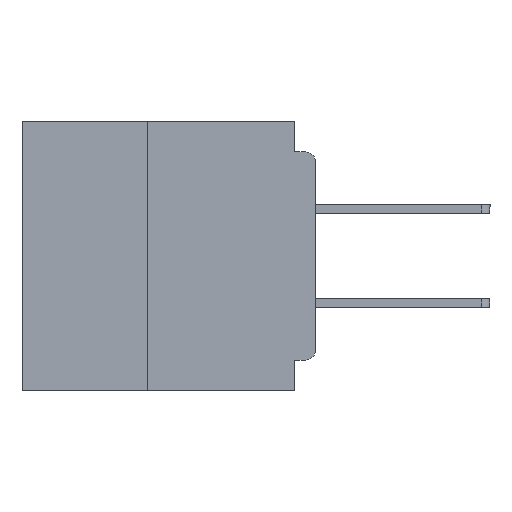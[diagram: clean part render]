
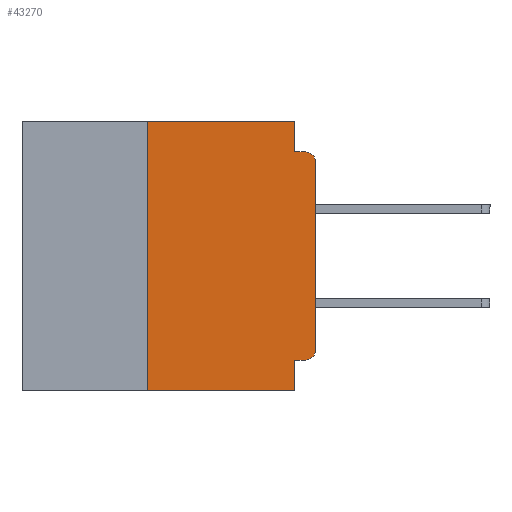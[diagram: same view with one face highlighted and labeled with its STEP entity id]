
A CAD part, left-side view. The second image highlights one B-rep face of the part: STEP entity #43270.
In plain terms, the highlighted planar face has unit normal (-1, 0, 0).
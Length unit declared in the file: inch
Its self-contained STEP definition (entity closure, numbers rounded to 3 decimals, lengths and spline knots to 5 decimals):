
#7 = DIRECTION ( 'NONE',  ( 0., 0., -1. ) ) ;
#875 = ORIENTED_EDGE ( 'NONE', *, *, #9050, .F. ) ;
#1804 = VERTEX_POINT ( 'NONE', #47177 ) ;
#3083 = VECTOR ( 'NONE', #30491, 39.37008 ) ;
#5957 = LINE ( 'NONE', #28612, #47334 ) ;
#6154 = EDGE_CURVE ( 'NONE', #41507, #40093, #37700, .T. ) ;
#6359 = CIRCLE ( 'NONE', #14164, 0.015 ) ;
#7134 = DIRECTION ( 'NONE',  ( 0., 0., -1. ) ) ;
#7153 = VERTEX_POINT ( 'NONE', #8263 ) ;
#7158 = VERTEX_POINT ( 'NONE', #48114 ) ;
#8028 = ORIENTED_EDGE ( 'NONE', *, *, #49835, .F. ) ;
#8263 = CARTESIAN_POINT ( 'NONE',  ( 0., 0.25, 0. ) ) ;
#9050 = EDGE_CURVE ( 'NONE', #7153, #45979, #5957, .T. ) ;
#9254 = DIRECTION ( 'NONE',  ( 0., 0., -1. ) ) ;
#9434 = VERTEX_POINT ( 'NONE', #19003 ) ;
#10384 = EDGE_CURVE ( 'NONE', #1804, #17054, #40367, .T. ) ;
#14164 = AXIS2_PLACEMENT_3D ( 'NONE', #15450, #43354, #19505 ) ;
#15142 = VERTEX_POINT ( 'NONE', #19496 ) ;
#15450 = CARTESIAN_POINT ( 'NONE',  ( 0., 0.015, -0.06 ) ) ;
#15528 = DIRECTION ( 'NONE',  ( 0., 1., 0. ) ) ;
#15632 = EDGE_CURVE ( 'NONE', #9434, #7153, #47252, .T. ) ;
#15823 = CARTESIAN_POINT ( 'NONE',  ( 0., 0.437, 0. ) ) ;
#17054 = VERTEX_POINT ( 'NONE', #35353 ) ;
#19003 = CARTESIAN_POINT ( 'NONE',  ( 0., 0.25, -0.4 ) ) ;
#19496 = CARTESIAN_POINT ( 'NONE',  ( 0., 0., -0.06 ) ) ;
#19505 = DIRECTION ( 'NONE',  ( 0., 0., -1. ) ) ;
#19951 = ORIENTED_EDGE ( 'NONE', *, *, #6154, .F. ) ;
#21781 = CARTESIAN_POINT ( 'NONE',  ( 0., 0.031, 0. ) ) ;
#21836 = EDGE_CURVE ( 'NONE', #7158, #41507, #35572, .T. ) ;
#22047 = CARTESIAN_POINT ( 'NONE',  ( 0., 0.437, -0.4 ) ) ;
#23594 = CARTESIAN_POINT ( 'NONE',  ( 0., 0., -0.355 ) ) ;
#23730 = VECTOR ( 'NONE', #15528, 39.37008 ) ;
#23887 = PLANE ( 'NONE',  #36084 ) ;
#24064 = VECTOR ( 'NONE', #7134, 39.37008 ) ;
#24315 = DIRECTION ( 'NONE',  ( 0., -1., 0. ) ) ;
#24422 = DIRECTION ( 'NONE',  ( -1., 0., 0. ) ) ;
#25305 = LINE ( 'NONE', #35236, #24064 ) ;
#25726 = EDGE_CURVE ( 'NONE', #15142, #17054, #6359, .T. ) ;
#26126 = EDGE_CURVE ( 'NONE', #9434, #40093, #38333, .T. ) ;
#27735 = AXIS2_PLACEMENT_3D ( 'NONE', #48212, #24422, #7 ) ;
#27854 = FACE_OUTER_BOUND ( 'NONE', #28532, .T. ) ;
#27897 = DIRECTION ( 'NONE',  ( 0., 0., -1. ) ) ;
#28532 = EDGE_LOOP ( 'NONE', ( #35690, #46757, #47830, #8028, #875, #38854, #29120, #19951, #34632, #43169 ) ) ;
#28612 = CARTESIAN_POINT ( 'NONE',  ( 0., 0.437, 0. ) ) ;
#28978 = VECTOR ( 'NONE', #49837, 39.37008 ) ;
#29120 = ORIENTED_EDGE ( 'NONE', *, *, #26126, .T. ) ;
#29752 = VECTOR ( 'NONE', #24315, 39.37008 ) ;
#30491 = DIRECTION ( 'NONE',  ( 0., 0., 1. ) ) ;
#33297 = CARTESIAN_POINT ( 'NONE',  ( 0., 0.031, -0.355 ) ) ;
#34283 = CARTESIAN_POINT ( 'NONE',  ( 0., 0., -0.34 ) ) ;
#34632 = ORIENTED_EDGE ( 'NONE', *, *, #21836, .F. ) ;
#35236 = CARTESIAN_POINT ( 'NONE',  ( 0., 0.031, 0. ) ) ;
#35274 = LINE ( 'NONE', #38345, #3083 ) ;
#35353 = CARTESIAN_POINT ( 'NONE',  ( 0., 0.015, -0.045 ) ) ;
#35572 = LINE ( 'NONE', #23594, #23730 ) ;
#35690 = ORIENTED_EDGE ( 'NONE', *, *, #36722, .T. ) ;
#35707 = CIRCLE ( 'NONE', #27735, 0.015 ) ;
#36084 = AXIS2_PLACEMENT_3D ( 'NONE', #15823, #51589, #27897 ) ;
#36722 = EDGE_CURVE ( 'NONE', #43676, #15142, #35274, .T. ) ;
#37070 = CARTESIAN_POINT ( 'NONE',  ( 0., 0.031, -0.4 ) ) ;
#37272 = CARTESIAN_POINT ( 'NONE',  ( 0., 0.031, -0.4 ) ) ;
#37700 = LINE ( 'NONE', #37272, #48251 ) ;
#38333 = LINE ( 'NONE', #22047, #28978 ) ;
#38345 = CARTESIAN_POINT ( 'NONE',  ( 0., 0., 0. ) ) ;
#38854 = ORIENTED_EDGE ( 'NONE', *, *, #15632, .F. ) ;
#40093 = VERTEX_POINT ( 'NONE', #37070 ) ;
#40367 = LINE ( 'NONE', #48110, #29752 ) ;
#41507 = VERTEX_POINT ( 'NONE', #33297 ) ;
#42237 = CARTESIAN_POINT ( 'NONE',  ( 0., 0.25, -0.4 ) ) ;
#43169 = ORIENTED_EDGE ( 'NONE', *, *, #51538, .T. ) ;
#43270 = ADVANCED_FACE ( 'NONE', ( #27854 ), #23887, .F. ) ;
#43354 = DIRECTION ( 'NONE',  ( -1., 0., 0. ) ) ;
#43676 = VERTEX_POINT ( 'NONE', #34283 ) ;
#44457 = DIRECTION ( 'NONE',  ( 0., -1., 0. ) ) ;
#45979 = VERTEX_POINT ( 'NONE', #21781 ) ;
#46003 = VECTOR ( 'NONE', #46217, 39.37008 ) ;
#46217 = DIRECTION ( 'NONE',  ( 0., 0., 1. ) ) ;
#46757 = ORIENTED_EDGE ( 'NONE', *, *, #25726, .T. ) ;
#47177 = CARTESIAN_POINT ( 'NONE',  ( 0., 0.031, -0.045 ) ) ;
#47252 = LINE ( 'NONE', #42237, #46003 ) ;
#47334 = VECTOR ( 'NONE', #44457, 39.37008 ) ;
#47830 = ORIENTED_EDGE ( 'NONE', *, *, #10384, .F. ) ;
#48110 = CARTESIAN_POINT ( 'NONE',  ( 0., 0., -0.045 ) ) ;
#48114 = CARTESIAN_POINT ( 'NONE',  ( 0., 0.015, -0.355 ) ) ;
#48212 = CARTESIAN_POINT ( 'NONE',  ( 0., 0.015, -0.34 ) ) ;
#48251 = VECTOR ( 'NONE', #9254, 39.37008 ) ;
#49835 = EDGE_CURVE ( 'NONE', #45979, #1804, #25305, .T. ) ;
#49837 = DIRECTION ( 'NONE',  ( 0., -1., 0. ) ) ;
#51538 = EDGE_CURVE ( 'NONE', #7158, #43676, #35707, .T. ) ;
#51589 = DIRECTION ( 'NONE',  ( 1., 0., 0. ) ) ;
